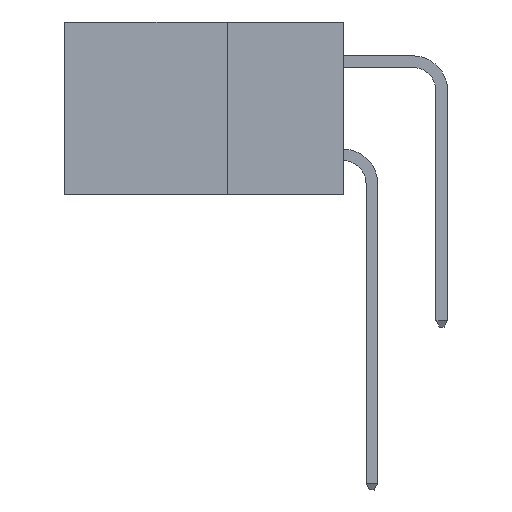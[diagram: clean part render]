
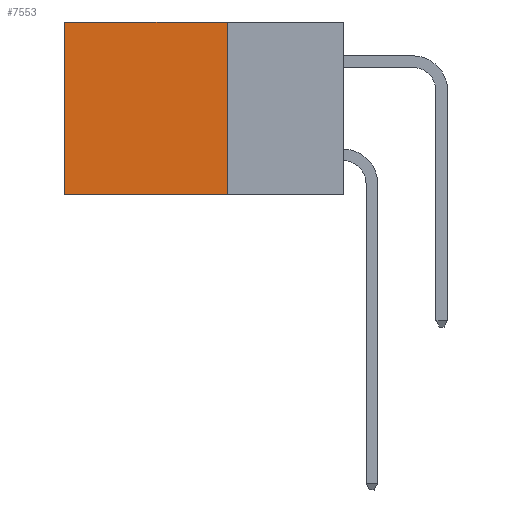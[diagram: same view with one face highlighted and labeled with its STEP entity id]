
A CAD part, left-side view. The second image highlights one B-rep face of the part: STEP entity #7553.
In plain terms, the highlighted planar face has unit normal (-1, 0, 0).
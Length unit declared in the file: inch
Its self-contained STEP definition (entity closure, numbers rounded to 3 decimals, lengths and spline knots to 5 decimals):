
#993 = CARTESIAN_POINT ( 'NONE',  ( 0.298, 0.25, 0. ) ) ;
#2349 = DIRECTION ( 'NONE',  ( 0., 1., 0. ) ) ;
#4012 = VECTOR ( 'NONE', #23857, 39.37008 ) ;
#5706 = LINE ( 'NONE', #28405, #18314 ) ;
#5815 = PLANE ( 'NONE',  #21913 ) ;
#5995 = ORIENTED_EDGE ( 'NONE', *, *, #24112, .F. ) ;
#6880 = EDGE_CURVE ( 'NONE', #9977, #21971, #25602, .T. ) ;
#7461 = CARTESIAN_POINT ( 'NONE',  ( 0.298, 0.25, 0. ) ) ;
#7553 = ADVANCED_FACE ( 'NONE', ( #12814 ), #5815, .F. ) ;
#8167 = CARTESIAN_POINT ( 'NONE',  ( 0.298, 0.25, -0.37 ) ) ;
#8258 = DIRECTION ( 'NONE',  ( 1., 0., 0. ) ) ;
#9977 = VERTEX_POINT ( 'NONE', #993 ) ;
#12509 = CARTESIAN_POINT ( 'NONE',  ( 0.298, 0.25, -0.37 ) ) ;
#12814 = FACE_OUTER_BOUND ( 'NONE', #26355, .T. ) ;
#14506 = DIRECTION ( 'NONE',  ( 0., 0., -1. ) ) ;
#15194 = LINE ( 'NONE', #7461, #4012 ) ;
#17134 = CARTESIAN_POINT ( 'NONE',  ( 0.298, 0.6, -0.37 ) ) ;
#17410 = VERTEX_POINT ( 'NONE', #8167 ) ;
#18314 = VECTOR ( 'NONE', #14506, 39.37008 ) ;
#19872 = ORIENTED_EDGE ( 'NONE', *, *, #26032, .F. ) ;
#20048 = VECTOR ( 'NONE', #2349, 39.37008 ) ;
#20519 = EDGE_CURVE ( 'NONE', #21971, #29666, #5706, .T. ) ;
#21021 = ORIENTED_EDGE ( 'NONE', *, *, #6880, .T. ) ;
#21913 = AXIS2_PLACEMENT_3D ( 'NONE', #22282, #8258, #24608 ) ;
#21971 = VERTEX_POINT ( 'NONE', #29426 ) ;
#22282 = CARTESIAN_POINT ( 'NONE',  ( 0.298, 0.25, 0. ) ) ;
#23857 = DIRECTION ( 'NONE',  ( 0., 0., -1. ) ) ;
#24112 = EDGE_CURVE ( 'NONE', #17410, #29666, #24755, .T. ) ;
#24608 = DIRECTION ( 'NONE',  ( 0., 0., -1. ) ) ;
#24641 = DIRECTION ( 'NONE',  ( 0., 1., 0. ) ) ;
#24755 = LINE ( 'NONE', #12509, #20048 ) ;
#24866 = VECTOR ( 'NONE', #24641, 39.37008 ) ;
#25602 = LINE ( 'NONE', #26981, #24866 ) ;
#26032 = EDGE_CURVE ( 'NONE', #9977, #17410, #15194, .T. ) ;
#26274 = ORIENTED_EDGE ( 'NONE', *, *, #20519, .T. ) ;
#26355 = EDGE_LOOP ( 'NONE', ( #26274, #5995, #19872, #21021 ) ) ;
#26981 = CARTESIAN_POINT ( 'NONE',  ( 0.298, 0.25, 0. ) ) ;
#28405 = CARTESIAN_POINT ( 'NONE',  ( 0.298, 0.6, 0. ) ) ;
#29426 = CARTESIAN_POINT ( 'NONE',  ( 0.298, 0.6, 0. ) ) ;
#29666 = VERTEX_POINT ( 'NONE', #17134 ) ;
